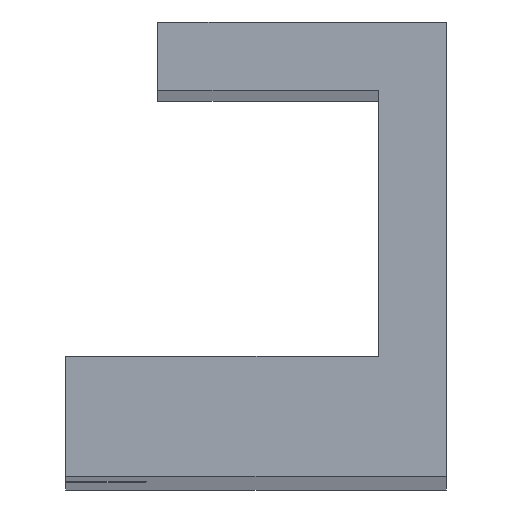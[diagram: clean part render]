
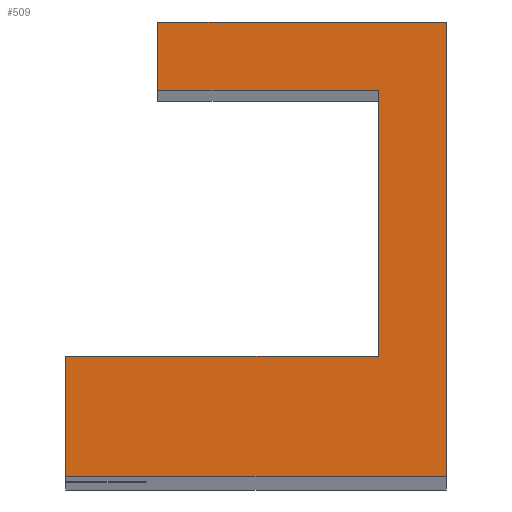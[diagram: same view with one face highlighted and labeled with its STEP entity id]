
A CAD part, top view. The second image highlights one B-rep face of the part: STEP entity #509.
In plain terms, the highlighted planar face has unit normal (0, 0, 1).
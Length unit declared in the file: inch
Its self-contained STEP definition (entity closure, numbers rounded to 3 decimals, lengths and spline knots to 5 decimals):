
#75=FACE_OUTER_BOUND('',#106,.T.);
#106=EDGE_LOOP('',(#408,#409,#410,#411,#412,#413,#414,#415));
#130=LINE('',#744,#177);
#133=LINE('',#749,#180);
#135=LINE('',#754,#182);
#141=LINE('',#782,#188);
#151=LINE('',#802,#198);
#159=LINE('',#816,#206);
#161=LINE('',#822,#208);
#162=LINE('',#823,#209);
#177=VECTOR('',#598,0.3937);
#180=VECTOR('',#603,0.3937);
#182=VECTOR('',#607,0.3937);
#188=VECTOR('',#631,0.3937);
#198=VECTOR('',#647,0.3937);
#206=VECTOR('',#659,0.3937);
#208=VECTOR('',#667,0.3937);
#209=VECTOR('',#668,0.3937);
#223=VERTEX_POINT('',#741);
#224=VERTEX_POINT('',#743);
#225=VERTEX_POINT('',#747);
#227=VERTEX_POINT('',#752);
#238=VERTEX_POINT('',#776);
#240=VERTEX_POINT('',#780);
#247=VERTEX_POINT('',#800);
#252=VERTEX_POINT('',#821);
#274=EDGE_CURVE('',#223,#224,#130,.T.);
#277=EDGE_CURVE('',#225,#223,#133,.T.);
#279=EDGE_CURVE('',#227,#225,#135,.T.);
#293=EDGE_CURVE('',#238,#240,#141,.T.);
#303=EDGE_CURVE('',#247,#240,#151,.T.);
#311=EDGE_CURVE('',#238,#227,#159,.T.);
#313=EDGE_CURVE('',#252,#247,#161,.T.);
#314=EDGE_CURVE('',#224,#252,#162,.T.);
#408=ORIENTED_EDGE('',*,*,#293,.T.);
#409=ORIENTED_EDGE('',*,*,#303,.F.);
#410=ORIENTED_EDGE('',*,*,#313,.F.);
#411=ORIENTED_EDGE('',*,*,#314,.F.);
#412=ORIENTED_EDGE('',*,*,#274,.F.);
#413=ORIENTED_EDGE('',*,*,#277,.F.);
#414=ORIENTED_EDGE('',*,*,#279,.F.);
#415=ORIENTED_EDGE('',*,*,#311,.F.);
#494=PLANE('',#560);
#509=ADVANCED_FACE('',(#75),#494,.F.);
#560=AXIS2_PLACEMENT_3D('',#820,#665,#666);
#598=DIRECTION('',(0.,1.,0.));
#603=DIRECTION('',(-1.,0.,0.));
#607=DIRECTION('',(0.,1.,0.));
#631=DIRECTION('',(0.,-1.,0.));
#647=DIRECTION('',(-1.,0.,0.));
#659=DIRECTION('',(1.,0.,0.));
#665=DIRECTION('center_axis',(0.,0.,-1.));
#666=DIRECTION('ref_axis',(-1.,0.,0.));
#667=DIRECTION('',(0.,-1.,0.));
#668=DIRECTION('',(1.,0.,0.));
#741=CARTESIAN_POINT('',(0.13,0.33465,6.80194));
#743=CARTESIAN_POINT('',(0.13,0.3937,6.80194));
#744=CARTESIAN_POINT('',(0.13,0.26575,6.80194));
#747=CARTESIAN_POINT('',(0.32094,0.33465,6.80194));
#749=CARTESIAN_POINT('',(0.145,0.33465,6.80194));
#752=CARTESIAN_POINT('',(0.32094,0.10406,6.80194));
#754=CARTESIAN_POINT('',(0.32094,0.26575,6.80194));
#776=CARTESIAN_POINT('',(0.05,0.10406,6.80194));
#780=CARTESIAN_POINT('',(0.05,0.,6.80194));
#782=CARTESIAN_POINT('',(0.05,0.1305,6.80194));
#800=CARTESIAN_POINT('',(0.38,0.,6.80194));
#802=CARTESIAN_POINT('',(0.095,0.,6.80194));
#816=CARTESIAN_POINT('',(0.,0.10406,6.80194));
#820=CARTESIAN_POINT('Origin',(0.19,0.19685,6.80194));
#821=CARTESIAN_POINT('',(0.38,0.3937,6.80194));
#822=CARTESIAN_POINT('',(0.38,0.09843,6.80194));
#823=CARTESIAN_POINT('',(0.285,0.3937,6.80194));
